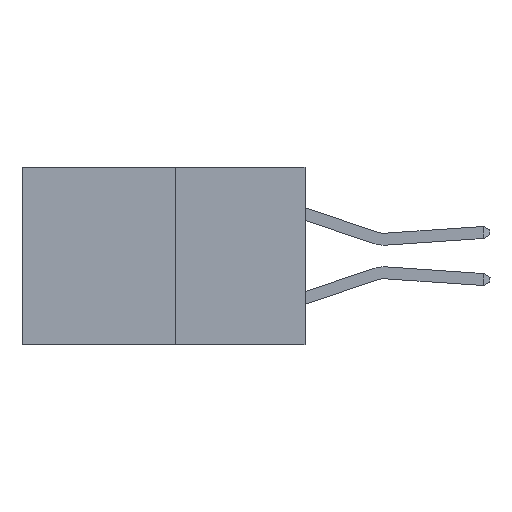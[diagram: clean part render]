
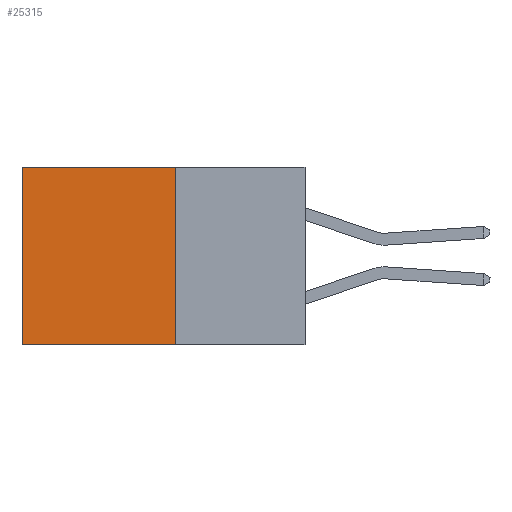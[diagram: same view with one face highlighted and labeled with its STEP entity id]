
A CAD part, left-side view. The second image highlights one B-rep face of the part: STEP entity #25315.
In plain terms, the highlighted planar face has unit normal (-1, 0, 0).
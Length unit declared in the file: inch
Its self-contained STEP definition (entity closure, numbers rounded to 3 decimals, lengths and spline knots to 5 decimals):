
#874 = DIRECTION ( 'NONE',  ( 1., 0., 0. ) ) ;
#1234 = CARTESIAN_POINT ( 'NONE',  ( 0.277, 0.27, -0.37 ) ) ;
#3093 = CARTESIAN_POINT ( 'NONE',  ( 0.277, 0.27, 0. ) ) ;
#3857 = CARTESIAN_POINT ( 'NONE',  ( 0.277, 0.27, 0. ) ) ;
#4725 = CARTESIAN_POINT ( 'NONE',  ( 0.277, 0.59, -0.37 ) ) ;
#5583 = LINE ( 'NONE', #19766, #10516 ) ;
#6169 = ORIENTED_EDGE ( 'NONE', *, *, #14570, .F. ) ;
#6310 = DIRECTION ( 'NONE',  ( 0., 1., 0. ) ) ;
#6617 = VERTEX_POINT ( 'NONE', #1234 ) ;
#8700 = LINE ( 'NONE', #22781, #20785 ) ;
#9631 = DIRECTION ( 'NONE',  ( 0., 0., -1. ) ) ;
#9877 = LINE ( 'NONE', #4725, #21931 ) ;
#9997 = VERTEX_POINT ( 'NONE', #27857 ) ;
#10516 = VECTOR ( 'NONE', #22186, 39.37008 ) ;
#11525 = ORIENTED_EDGE ( 'NONE', *, *, #18380, .T. ) ;
#13001 = PLANE ( 'NONE',  #16061 ) ;
#13370 = CARTESIAN_POINT ( 'NONE',  ( 0.277, 0.59, 0. ) ) ;
#14570 = EDGE_CURVE ( 'NONE', #6617, #9997, #5583, .T. ) ;
#15386 = CARTESIAN_POINT ( 'NONE',  ( 0.277, 0.27, -0.37 ) ) ;
#16061 = AXIS2_PLACEMENT_3D ( 'NONE', #15386, #874, #17788 ) ;
#16304 = LINE ( 'NONE', #3857, #28284 ) ;
#17788 = DIRECTION ( 'NONE',  ( 0., 0., -1. ) ) ;
#18380 = EDGE_CURVE ( 'NONE', #26008, #9997, #9877, .T. ) ;
#19766 = CARTESIAN_POINT ( 'NONE',  ( 0.277, 0.27, -0.37 ) ) ;
#20200 = ORIENTED_EDGE ( 'NONE', *, *, #23370, .F. ) ;
#20371 = DIRECTION ( 'NONE',  ( 0., 0., -1. ) ) ;
#20785 = VECTOR ( 'NONE', #20371, 39.37008 ) ;
#21931 = VECTOR ( 'NONE', #9631, 39.37008 ) ;
#22186 = DIRECTION ( 'NONE',  ( 0., 1., 0. ) ) ;
#22781 = CARTESIAN_POINT ( 'NONE',  ( 0.277, 0.27, -0.37 ) ) ;
#23271 = FACE_OUTER_BOUND ( 'NONE', #25531, .T. ) ;
#23370 = EDGE_CURVE ( 'NONE', #27209, #6617, #8700, .T. ) ;
#24508 = ORIENTED_EDGE ( 'NONE', *, *, #26764, .T. ) ;
#25315 = ADVANCED_FACE ( 'NONE', ( #23271 ), #13001, .F. ) ;
#25531 = EDGE_LOOP ( 'NONE', ( #11525, #6169, #20200, #24508 ) ) ;
#26008 = VERTEX_POINT ( 'NONE', #13370 ) ;
#26764 = EDGE_CURVE ( 'NONE', #27209, #26008, #16304, .T. ) ;
#27209 = VERTEX_POINT ( 'NONE', #3093 ) ;
#27857 = CARTESIAN_POINT ( 'NONE',  ( 0.277, 0.59, -0.37 ) ) ;
#28284 = VECTOR ( 'NONE', #6310, 39.37008 ) ;
